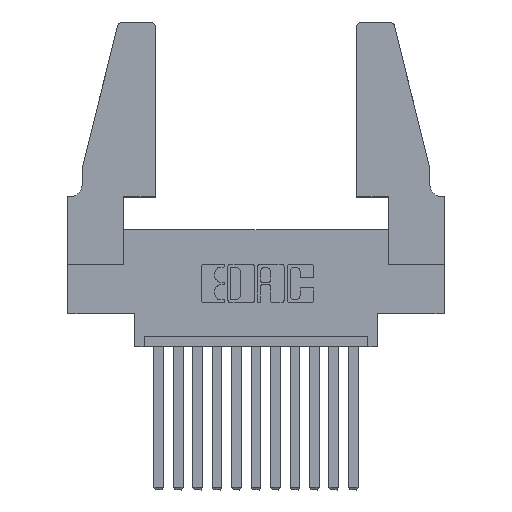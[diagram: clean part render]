
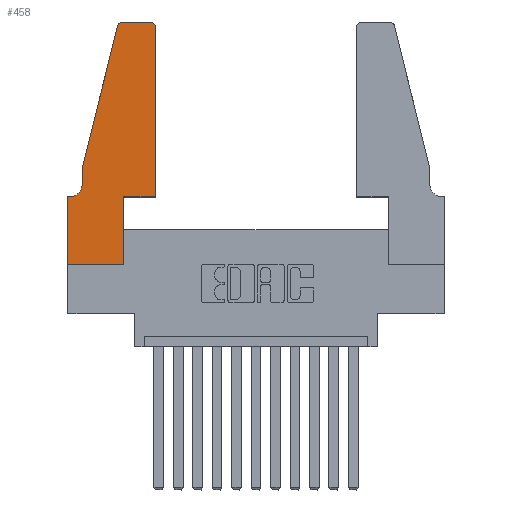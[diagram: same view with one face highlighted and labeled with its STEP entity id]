
A CAD part, top view. The second image highlights one B-rep face of the part: STEP entity #458.
In plain terms, the highlighted planar face has unit normal (0, 0, 1).
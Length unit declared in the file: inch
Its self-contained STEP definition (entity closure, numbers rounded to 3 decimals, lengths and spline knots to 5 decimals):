
#129 = CARTESIAN_POINT ( 'NONE',  ( 0., 0., 0.37 ) ) ;
#178 = VERTEX_POINT ( 'NONE', #10474 ) ;
#458 = ADVANCED_FACE ( 'NONE', ( #7126 ), #10769, .T. ) ;
#519 = EDGE_CURVE ( 'NONE', #14194, #13937, #2072, .T. ) ;
#643 = EDGE_CURVE ( 'NONE', #8918, #5586, #823, .T. ) ;
#663 = VERTEX_POINT ( 'NONE', #2100 ) ;
#823 = LINE ( 'NONE', #1742, #13993 ) ;
#896 = DIRECTION ( 'NONE',  ( -0.239, -0.971, 0. ) ) ;
#1665 = VECTOR ( 'NONE', #11354, 39.37008 ) ;
#1719 = DIRECTION ( 'NONE',  ( 1., 0., 0. ) ) ;
#1742 = CARTESIAN_POINT ( 'NONE',  ( 0.4505, 0.35, 0.37 ) ) ;
#1801 = LINE ( 'NONE', #13741, #7369 ) ;
#1945 = CARTESIAN_POINT ( 'NONE',  ( 0.0755, 0.5, 0.37 ) ) ;
#2009 = ORIENTED_EDGE ( 'NONE', *, *, #8692, .T. ) ;
#2072 = LINE ( 'NONE', #1945, #9937 ) ;
#2100 = CARTESIAN_POINT ( 'NONE',  ( 0.4505, 1.22, 0.37 ) ) ;
#2202 = ORIENTED_EDGE ( 'NONE', *, *, #8412, .T. ) ;
#2209 = CARTESIAN_POINT ( 'NONE',  ( 0.2865, 0., 0.37 ) ) ;
#2270 = VECTOR ( 'NONE', #2421, 39.37008 ) ;
#2305 = VERTEX_POINT ( 'NONE', #3647 ) ;
#2312 = CARTESIAN_POINT ( 'NONE',  ( 0.284, 1.22, 0.37 ) ) ;
#2421 = DIRECTION ( 'NONE',  ( 1., 0., 0. ) ) ;
#2697 = EDGE_CURVE ( 'NONE', #12665, #8918, #9696, .T. ) ;
#2815 = CARTESIAN_POINT ( 'NONE',  ( 0.2865, 0.35, 0.37 ) ) ;
#2876 = DIRECTION ( 'NONE',  ( 0., 0., 1. ) ) ;
#3020 = LINE ( 'NONE', #13278, #8407 ) ;
#3126 = AXIS2_PLACEMENT_3D ( 'NONE', #13963, #14007, #1719 ) ;
#3132 = CARTESIAN_POINT ( 'NONE',  ( 0.284, 1.25, 0.37 ) ) ;
#3164 = CARTESIAN_POINT ( 'NONE',  ( 0.25487, 1.22718, 0.37 ) ) ;
#3229 = LINE ( 'NONE', #11410, #1665 ) ;
#3241 = VECTOR ( 'NONE', #3997, 39.37008 ) ;
#3432 = DIRECTION ( 'NONE',  ( 1., 0., 0. ) ) ;
#3647 = CARTESIAN_POINT ( 'NONE',  ( 0.0055, 0.35, 0.37 ) ) ;
#3690 = ORIENTED_EDGE ( 'NONE', *, *, #6152, .T. ) ;
#3817 = CARTESIAN_POINT ( 'NONE',  ( 0.4205, 1.25, 0.37 ) ) ;
#3962 = CIRCLE ( 'NONE', #6258, 0.03 ) ;
#3997 = DIRECTION ( 'NONE',  ( 0., 1., 0. ) ) ;
#4137 = ORIENTED_EDGE ( 'NONE', *, *, #11775, .T. ) ;
#4486 = CARTESIAN_POINT ( 'NONE',  ( 0.4505, 0.35, 0.37 ) ) ;
#4542 = CIRCLE ( 'NONE', #8592, 0.07 ) ;
#4910 = CARTESIAN_POINT ( 'NONE',  ( 0.0755, 0.5, 0.37 ) ) ;
#5094 = VECTOR ( 'NONE', #7602, 39.37008 ) ;
#5147 = CARTESIAN_POINT ( 'NONE',  ( 0.0055, 0.42, 0.37 ) ) ;
#5233 = DIRECTION ( 'NONE',  ( -1., 0., 0. ) ) ;
#5411 = AXIS2_PLACEMENT_3D ( 'NONE', #13853, #2876, #8427 ) ;
#5586 = VERTEX_POINT ( 'NONE', #4486 ) ;
#5769 = CARTESIAN_POINT ( 'NONE',  ( 0.2605, 1.25, 0.37 ) ) ;
#6152 = EDGE_CURVE ( 'NONE', #663, #13957, #14087, .T. ) ;
#6258 = AXIS2_PLACEMENT_3D ( 'NONE', #2312, #7796, #3432 ) ;
#6274 = LINE ( 'NONE', #129, #2270 ) ;
#6546 = ORIENTED_EDGE ( 'NONE', *, *, #9983, .T. ) ;
#7085 = DIRECTION ( 'NONE',  ( 0., -1., 0. ) ) ;
#7126 = FACE_OUTER_BOUND ( 'NONE', #9145, .T. ) ;
#7369 = VECTOR ( 'NONE', #7085, 39.37008 ) ;
#7602 = DIRECTION ( 'NONE',  ( 0., 1., 0. ) ) ;
#7654 = LINE ( 'NONE', #5769, #9280 ) ;
#7796 = DIRECTION ( 'NONE',  ( 0., 0., 1. ) ) ;
#7875 = EDGE_CURVE ( 'NONE', #7997, #2305, #4542, .T. ) ;
#7997 = VERTEX_POINT ( 'NONE', #8752 ) ;
#8053 = EDGE_CURVE ( 'NONE', #12695, #12665, #6274, .T. ) ;
#8407 = VECTOR ( 'NONE', #11191, 39.37008 ) ;
#8412 = EDGE_CURVE ( 'NONE', #13957, #13671, #7654, .T. ) ;
#8427 = DIRECTION ( 'NONE',  ( 1., 0., 0. ) ) ;
#8592 = AXIS2_PLACEMENT_3D ( 'NONE', #5147, #14147, #5233 ) ;
#8692 = EDGE_CURVE ( 'NONE', #13671, #14194, #3962, .T. ) ;
#8752 = CARTESIAN_POINT ( 'NONE',  ( 0.0755, 0.42, 0.37 ) ) ;
#8918 = VERTEX_POINT ( 'NONE', #9585 ) ;
#9145 = EDGE_LOOP ( 'NONE', ( #2202, #2009, #11794, #6546, #14058, #14162, #13649, #10546, #10678, #13855, #4137, #3690 ) ) ;
#9169 = LINE ( 'NONE', #9570, #5094 ) ;
#9280 = VECTOR ( 'NONE', #10448, 39.37008 ) ;
#9570 = CARTESIAN_POINT ( 'NONE',  ( 0.4505, 0.35, 0.37 ) ) ;
#9585 = CARTESIAN_POINT ( 'NONE',  ( 0.2865, 0.35, 0.37 ) ) ;
#9696 = LINE ( 'NONE', #2815, #3241 ) ;
#9937 = VECTOR ( 'NONE', #896, 39.37008 ) ;
#9983 = EDGE_CURVE ( 'NONE', #13937, #7997, #3020, .T. ) ;
#10373 = CARTESIAN_POINT ( 'NONE',  ( 0., 0., 0.37 ) ) ;
#10448 = DIRECTION ( 'NONE',  ( -1., 0., 0. ) ) ;
#10474 = CARTESIAN_POINT ( 'NONE',  ( 0., 0.35, 0.37 ) ) ;
#10546 = ORIENTED_EDGE ( 'NONE', *, *, #8053, .T. ) ;
#10678 = ORIENTED_EDGE ( 'NONE', *, *, #2697, .T. ) ;
#10769 = PLANE ( 'NONE',  #3126 ) ;
#10872 = EDGE_CURVE ( 'NONE', #2305, #178, #3229, .T. ) ;
#11191 = DIRECTION ( 'NONE',  ( 0., -1., 0. ) ) ;
#11354 = DIRECTION ( 'NONE',  ( -1., 0., 0. ) ) ;
#11410 = CARTESIAN_POINT ( 'NONE',  ( 0.0755, 0.35, 0.37 ) ) ;
#11775 = EDGE_CURVE ( 'NONE', #5586, #663, #9169, .T. ) ;
#11794 = ORIENTED_EDGE ( 'NONE', *, *, #519, .T. ) ;
#12216 = EDGE_CURVE ( 'NONE', #178, #12695, #1801, .T. ) ;
#12665 = VERTEX_POINT ( 'NONE', #2209 ) ;
#12695 = VERTEX_POINT ( 'NONE', #10373 ) ;
#13278 = CARTESIAN_POINT ( 'NONE',  ( 0.0755, 0.5, 0.37 ) ) ;
#13649 = ORIENTED_EDGE ( 'NONE', *, *, #12216, .T. ) ;
#13671 = VERTEX_POINT ( 'NONE', #3132 ) ;
#13741 = CARTESIAN_POINT ( 'NONE',  ( 0., 0., 0.37 ) ) ;
#13853 = CARTESIAN_POINT ( 'NONE',  ( 0.4205, 1.22, 0.37 ) ) ;
#13855 = ORIENTED_EDGE ( 'NONE', *, *, #643, .T. ) ;
#13937 = VERTEX_POINT ( 'NONE', #4910 ) ;
#13957 = VERTEX_POINT ( 'NONE', #3817 ) ;
#13963 = CARTESIAN_POINT ( 'NONE',  ( 0., 0.35, 0.37 ) ) ;
#13993 = VECTOR ( 'NONE', #14504, 39.37008 ) ;
#14007 = DIRECTION ( 'NONE',  ( 0., 0., 1. ) ) ;
#14058 = ORIENTED_EDGE ( 'NONE', *, *, #7875, .T. ) ;
#14087 = CIRCLE ( 'NONE', #5411, 0.03 ) ;
#14147 = DIRECTION ( 'NONE',  ( 0., 0., -1. ) ) ;
#14162 = ORIENTED_EDGE ( 'NONE', *, *, #10872, .T. ) ;
#14194 = VERTEX_POINT ( 'NONE', #3164 ) ;
#14504 = DIRECTION ( 'NONE',  ( 1., 0., 0. ) ) ;
